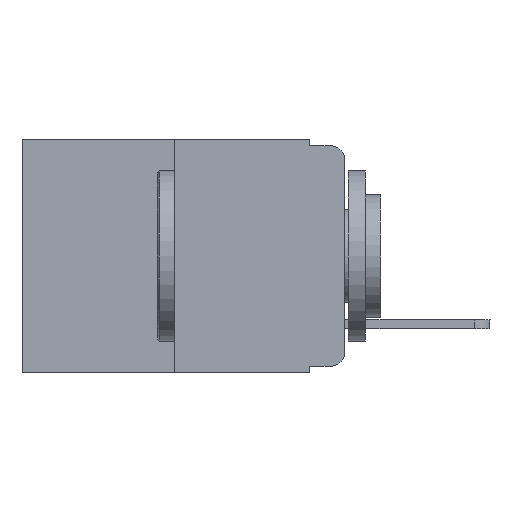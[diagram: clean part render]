
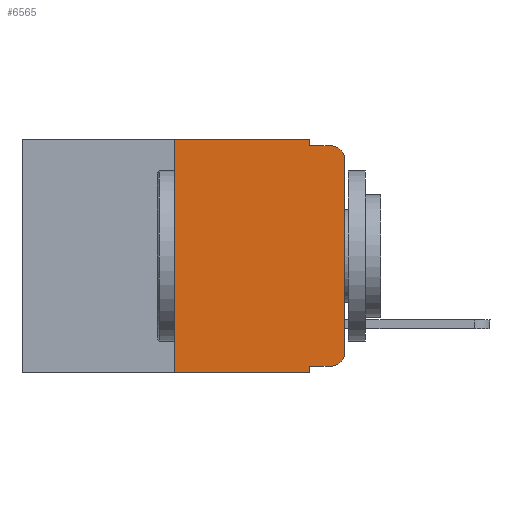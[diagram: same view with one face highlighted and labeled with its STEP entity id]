
A CAD part, left-side view. The second image highlights one B-rep face of the part: STEP entity #6565.
In plain terms, the highlighted planar face has unit normal (-1, 0, 0).
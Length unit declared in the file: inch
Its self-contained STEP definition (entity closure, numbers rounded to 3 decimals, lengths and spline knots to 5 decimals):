
#21 = CARTESIAN_POINT ( 'NONE',  ( 0., 0.25, -0.343 ) ) ;
#196 = LINE ( 'NONE', #14760, #16793 ) ;
#239 = VERTEX_POINT ( 'NONE', #14933 ) ;
#409 = DIRECTION ( 'NONE',  ( 0., -1., 0. ) ) ;
#1284 = CARTESIAN_POINT ( 'NONE',  ( 0., 0., -0.03 ) ) ;
#1312 = VERTEX_POINT ( 'NONE', #12193 ) ;
#1546 = CARTESIAN_POINT ( 'NONE',  ( 0., 0.051, -0.01 ) ) ;
#1997 = VECTOR ( 'NONE', #409, 39.37008 ) ;
#2019 = EDGE_CURVE ( 'NONE', #1312, #17011, #14768, .T. ) ;
#2156 = DIRECTION ( 'NONE',  ( 0., 0., -1. ) ) ;
#2348 = PLANE ( 'NONE',  #17111 ) ;
#2387 = CARTESIAN_POINT ( 'NONE',  ( 0., 0.02, -0.01 ) ) ;
#2548 = LINE ( 'NONE', #8341, #3277 ) ;
#2621 = VERTEX_POINT ( 'NONE', #1284 ) ;
#3041 = EDGE_CURVE ( 'NONE', #239, #1312, #2548, .T. ) ;
#3277 = VECTOR ( 'NONE', #14303, 39.37008 ) ;
#3289 = ORIENTED_EDGE ( 'NONE', *, *, #11555, .F. ) ;
#3496 = LINE ( 'NONE', #9273, #12115 ) ;
#3513 = FACE_OUTER_BOUND ( 'NONE', #3634, .T. ) ;
#3575 = AXIS2_PLACEMENT_3D ( 'NONE', #3685, #9278, #15057 ) ;
#3634 = EDGE_LOOP ( 'NONE', ( #9910, #13635, #5944, #3289, #17472, #13416, #10478, #5848, #12055, #5691 ) ) ;
#3653 = CARTESIAN_POINT ( 'NONE',  ( 0., 0.473, 0. ) ) ;
#3685 = CARTESIAN_POINT ( 'NONE',  ( 0., 0.02, -0.313 ) ) ;
#3775 = CARTESIAN_POINT ( 'NONE',  ( 0., 0.473, 0. ) ) ;
#4214 = CARTESIAN_POINT ( 'NONE',  ( 0., 0.02, -0.03 ) ) ;
#4606 = LINE ( 'NONE', #10377, #15529 ) ;
#4791 = EDGE_CURVE ( 'NONE', #17011, #2621, #196, .T. ) ;
#4880 = DIRECTION ( 'NONE',  ( 0., 0., -1. ) ) ;
#5464 = EDGE_CURVE ( 'NONE', #11292, #9115, #4606, .T. ) ;
#5646 = EDGE_CURVE ( 'NONE', #239, #10570, #16512, .T. ) ;
#5670 = CARTESIAN_POINT ( 'NONE',  ( 0., 0.473, -0.343 ) ) ;
#5691 = ORIENTED_EDGE ( 'NONE', *, *, #2019, .T. ) ;
#5767 = VERTEX_POINT ( 'NONE', #2387 ) ;
#5848 = ORIENTED_EDGE ( 'NONE', *, *, #5646, .F. ) ;
#5944 = ORIENTED_EDGE ( 'NONE', *, *, #17841, .F. ) ;
#6565 = ADVANCED_FACE ( 'NONE', ( #3513 ), #2348, .F. ) ;
#6752 = CARTESIAN_POINT ( 'NONE',  ( 0., 0.051, -0.01 ) ) ;
#6867 = EDGE_CURVE ( 'NONE', #9115, #13952, #9330, .T. ) ;
#7043 = VERTEX_POINT ( 'NONE', #6752 ) ;
#7252 = CARTESIAN_POINT ( 'NONE',  ( 0., 0., -0.313 ) ) ;
#7463 = LINE ( 'NONE', #5670, #8075 ) ;
#7923 = EDGE_CURVE ( 'NONE', #11292, #10570, #7463, .T. ) ;
#8075 = VECTOR ( 'NONE', #14665, 39.37008 ) ;
#8132 = DIRECTION ( 'NONE',  ( 1., 0., 0. ) ) ;
#8341 = CARTESIAN_POINT ( 'NONE',  ( 0., 0.051, -0.333 ) ) ;
#8380 = DIRECTION ( 'NONE',  ( -1., 0., 0. ) ) ;
#8959 = DIRECTION ( 'NONE',  ( 0., 0., 1. ) ) ;
#9115 = VERTEX_POINT ( 'NONE', #9654 ) ;
#9237 = VECTOR ( 'NONE', #4880, 39.37008 ) ;
#9273 = CARTESIAN_POINT ( 'NONE',  ( 0., 0.051, 0. ) ) ;
#9278 = DIRECTION ( 'NONE',  ( -1., 0., 0. ) ) ;
#9330 = LINE ( 'NONE', #3653, #13195 ) ;
#9654 = CARTESIAN_POINT ( 'NONE',  ( 0., 0.25, 0. ) ) ;
#9910 = ORIENTED_EDGE ( 'NONE', *, *, #4791, .T. ) ;
#10283 = CARTESIAN_POINT ( 'NONE',  ( 0., 0.051, 0. ) ) ;
#10305 = DIRECTION ( 'NONE',  ( 0., 0., 1. ) ) ;
#10377 = CARTESIAN_POINT ( 'NONE',  ( 0., 0.25, 0. ) ) ;
#10478 = ORIENTED_EDGE ( 'NONE', *, *, #7923, .T. ) ;
#10570 = VERTEX_POINT ( 'NONE', #12755 ) ;
#11061 = AXIS2_PLACEMENT_3D ( 'NONE', #4214, #8380, #12819 ) ;
#11292 = VERTEX_POINT ( 'NONE', #21 ) ;
#11555 = EDGE_CURVE ( 'NONE', #13952, #7043, #3496, .T. ) ;
#12055 = ORIENTED_EDGE ( 'NONE', *, *, #3041, .T. ) ;
#12115 = VECTOR ( 'NONE', #2156, 39.37008 ) ;
#12193 = CARTESIAN_POINT ( 'NONE',  ( 0., 0.02, -0.333 ) ) ;
#12559 = CIRCLE ( 'NONE', #11061, 0.02 ) ;
#12755 = CARTESIAN_POINT ( 'NONE',  ( 0., 0.051, -0.343 ) ) ;
#12819 = DIRECTION ( 'NONE',  ( 0., 0., -1. ) ) ;
#13195 = VECTOR ( 'NONE', #14662, 39.37008 ) ;
#13416 = ORIENTED_EDGE ( 'NONE', *, *, #5464, .F. ) ;
#13635 = ORIENTED_EDGE ( 'NONE', *, *, #17387, .T. ) ;
#13952 = VERTEX_POINT ( 'NONE', #10283 ) ;
#13985 = DIRECTION ( 'NONE',  ( 0., 0., -1. ) ) ;
#14303 = DIRECTION ( 'NONE',  ( 0., -1., 0. ) ) ;
#14500 = LINE ( 'NONE', #1546, #1997 ) ;
#14662 = DIRECTION ( 'NONE',  ( 0., -1., 0. ) ) ;
#14665 = DIRECTION ( 'NONE',  ( 0., -1., 0. ) ) ;
#14760 = CARTESIAN_POINT ( 'NONE',  ( 0., 0., 0. ) ) ;
#14768 = CIRCLE ( 'NONE', #3575, 0.02 ) ;
#14933 = CARTESIAN_POINT ( 'NONE',  ( 0., 0.051, -0.333 ) ) ;
#15057 = DIRECTION ( 'NONE',  ( 0., 0., -1. ) ) ;
#15529 = VECTOR ( 'NONE', #8959, 39.37008 ) ;
#16512 = LINE ( 'NONE', #18125, #9237 ) ;
#16793 = VECTOR ( 'NONE', #10305, 39.37008 ) ;
#17011 = VERTEX_POINT ( 'NONE', #7252 ) ;
#17111 = AXIS2_PLACEMENT_3D ( 'NONE', #3775, #8132, #13985 ) ;
#17387 = EDGE_CURVE ( 'NONE', #2621, #5767, #12559, .T. ) ;
#17472 = ORIENTED_EDGE ( 'NONE', *, *, #6867, .F. ) ;
#17841 = EDGE_CURVE ( 'NONE', #7043, #5767, #14500, .T. ) ;
#18125 = CARTESIAN_POINT ( 'NONE',  ( 0., 0.051, 0. ) ) ;
